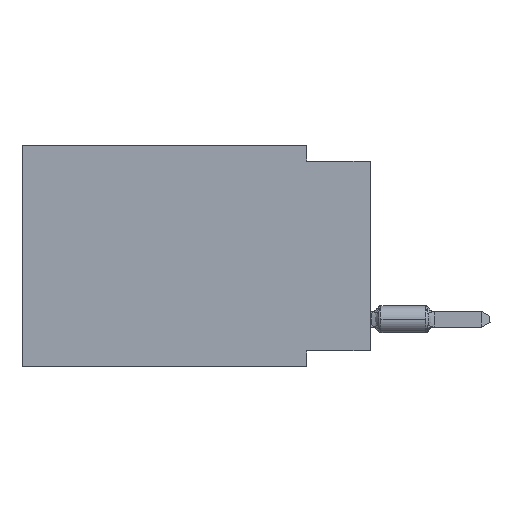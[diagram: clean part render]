
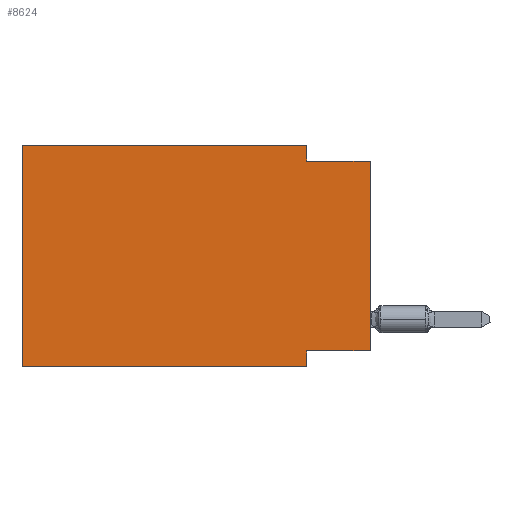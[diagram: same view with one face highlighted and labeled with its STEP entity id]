
A CAD part, left-side view. The second image highlights one B-rep face of the part: STEP entity #8624.
In plain terms, the highlighted planar face has unit normal (-1, 0, 0).
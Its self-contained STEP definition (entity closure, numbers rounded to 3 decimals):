
#944 = ORIENTED_EDGE ( 'NONE', *, *, #12527, .F. ) ;
#1265 = VERTEX_POINT ( 'NONE', #14624 ) ;
#1301 = CARTESIAN_POINT ( 'NONE',  ( 0., 0., -0.635 ) ) ;
#1429 = ORIENTED_EDGE ( 'NONE', *, *, #4571, .F. ) ;
#1516 = DIRECTION ( 'NONE',  ( 1., 0., 0. ) ) ;
#1956 = AXIS2_PLACEMENT_3D ( 'NONE', #15091, #1516, #2730 ) ;
#1975 = CARTESIAN_POINT ( 'NONE',  ( 0., 2.54, -8.89 ) ) ;
#2231 = DIRECTION ( 'NONE',  ( 0., -1., 0. ) ) ;
#2730 = DIRECTION ( 'NONE',  ( 0., 0., -1. ) ) ;
#2773 = VECTOR ( 'NONE', #16653, 1000. ) ;
#2868 = ORIENTED_EDGE ( 'NONE', *, *, #5183, .F. ) ;
#3701 = EDGE_LOOP ( 'NONE', ( #7441, #15460, #3800, #2868, #12337, #7311, #944, #1429 ) ) ;
#3723 = DIRECTION ( 'NONE',  ( 0., 0., 1. ) ) ;
#3760 = EDGE_CURVE ( 'NONE', #7027, #1265, #11920, .T. ) ;
#3800 = ORIENTED_EDGE ( 'NONE', *, *, #8189, .F. ) ;
#4400 = VERTEX_POINT ( 'NONE', #17971 ) ;
#4419 = CARTESIAN_POINT ( 'NONE',  ( 0., 13.97, 0. ) ) ;
#4571 = EDGE_CURVE ( 'NONE', #7027, #9537, #8265, .T. ) ;
#4629 = LINE ( 'NONE', #1975, #17296 ) ;
#4783 = VECTOR ( 'NONE', #3723, 1000. ) ;
#4808 = VERTEX_POINT ( 'NONE', #11140 ) ;
#5159 = LINE ( 'NONE', #8148, #8878 ) ;
#5183 = EDGE_CURVE ( 'NONE', #4808, #4400, #17662, .T. ) ;
#5289 = EDGE_CURVE ( 'NONE', #16948, #1265, #10808, .T. ) ;
#5504 = VECTOR ( 'NONE', #13842, 1000. ) ;
#5665 = DIRECTION ( 'NONE',  ( 0., 0., -1. ) ) ;
#6345 = CARTESIAN_POINT ( 'NONE',  ( 0., 0., -8.255 ) ) ;
#6824 = FACE_OUTER_BOUND ( 'NONE', #3701, .T. ) ;
#6937 = CARTESIAN_POINT ( 'NONE',  ( 0., 2.54, 0. ) ) ;
#7027 = VERTEX_POINT ( 'NONE', #6345 ) ;
#7311 = ORIENTED_EDGE ( 'NONE', *, *, #16249, .T. ) ;
#7441 = ORIENTED_EDGE ( 'NONE', *, *, #3760, .T. ) ;
#7714 = VECTOR ( 'NONE', #13861, 1000. ) ;
#7799 = VERTEX_POINT ( 'NONE', #11252 ) ;
#7800 = CARTESIAN_POINT ( 'NONE',  ( 0., 2.54, -8.89 ) ) ;
#8148 = CARTESIAN_POINT ( 'NONE',  ( 0., 13.97, -8.89 ) ) ;
#8189 = EDGE_CURVE ( 'NONE', #4400, #16948, #8214, .T. ) ;
#8214 = LINE ( 'NONE', #6937, #12452 ) ;
#8265 = LINE ( 'NONE', #14036, #7714 ) ;
#8624 = ADVANCED_FACE ( 'NONE', ( #6824 ), #14054, .F. ) ;
#8878 = VECTOR ( 'NONE', #16572, 1000. ) ;
#9163 = CARTESIAN_POINT ( 'NONE',  ( 0., 13.97, 0. ) ) ;
#9174 = CARTESIAN_POINT ( 'NONE',  ( 0., 0., 0. ) ) ;
#9513 = EDGE_CURVE ( 'NONE', #7799, #4808, #9889, .T. ) ;
#9537 = VERTEX_POINT ( 'NONE', #11349 ) ;
#9889 = LINE ( 'NONE', #4419, #5504 ) ;
#10203 = DIRECTION ( 'NONE',  ( 0., 0., -1. ) ) ;
#10808 = LINE ( 'NONE', #1301, #2773 ) ;
#11140 = CARTESIAN_POINT ( 'NONE',  ( 0., 13.97, 0. ) ) ;
#11252 = CARTESIAN_POINT ( 'NONE',  ( 0., 13.97, -8.89 ) ) ;
#11349 = CARTESIAN_POINT ( 'NONE',  ( 0., 2.54, -8.255 ) ) ;
#11920 = LINE ( 'NONE', #9174, #4783 ) ;
#12337 = ORIENTED_EDGE ( 'NONE', *, *, #9513, .F. ) ;
#12452 = VECTOR ( 'NONE', #5665, 1000. ) ;
#12527 = EDGE_CURVE ( 'NONE', #9537, #16989, #4629, .T. ) ;
#13842 = DIRECTION ( 'NONE',  ( 0., 0., 1. ) ) ;
#13861 = DIRECTION ( 'NONE',  ( 0., 1., 0. ) ) ;
#14036 = CARTESIAN_POINT ( 'NONE',  ( 0., 0., -8.255 ) ) ;
#14054 = PLANE ( 'NONE',  #1956 ) ;
#14154 = VECTOR ( 'NONE', #2231, 1000. ) ;
#14624 = CARTESIAN_POINT ( 'NONE',  ( 0., 0., -0.635 ) ) ;
#15091 = CARTESIAN_POINT ( 'NONE',  ( 0., 13.97, 0. ) ) ;
#15460 = ORIENTED_EDGE ( 'NONE', *, *, #5289, .F. ) ;
#16249 = EDGE_CURVE ( 'NONE', #7799, #16989, #5159, .T. ) ;
#16311 = CARTESIAN_POINT ( 'NONE',  ( 0., 2.54, -0.635 ) ) ;
#16572 = DIRECTION ( 'NONE',  ( 0., -1., 0. ) ) ;
#16653 = DIRECTION ( 'NONE',  ( 0., -1., 0. ) ) ;
#16948 = VERTEX_POINT ( 'NONE', #16311 ) ;
#16989 = VERTEX_POINT ( 'NONE', #7800 ) ;
#17296 = VECTOR ( 'NONE', #10203, 1000. ) ;
#17662 = LINE ( 'NONE', #9163, #14154 ) ;
#17971 = CARTESIAN_POINT ( 'NONE',  ( 0., 2.54, 0. ) ) ;
